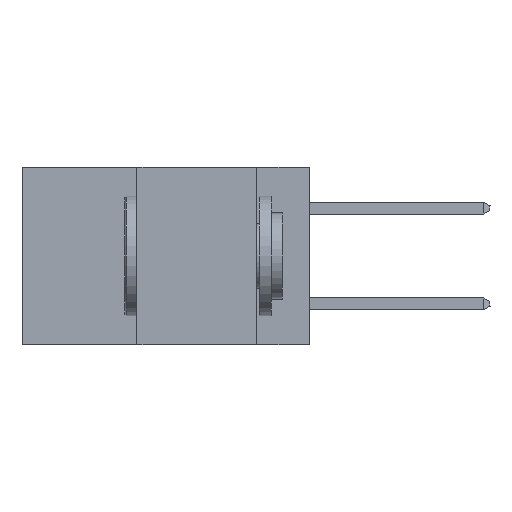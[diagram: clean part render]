
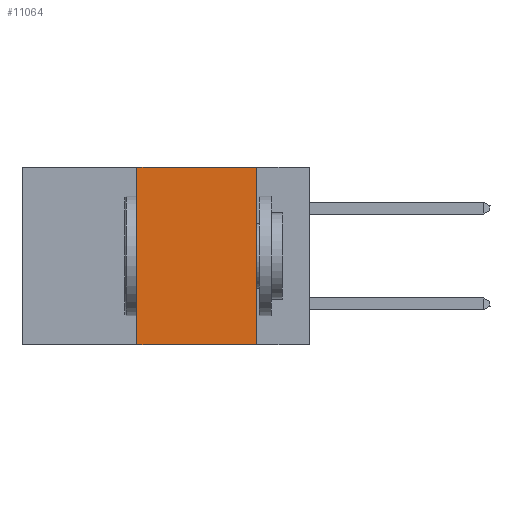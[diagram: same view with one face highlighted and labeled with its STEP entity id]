
A CAD part, left-side view. The second image highlights one B-rep face of the part: STEP entity #11064.
In plain terms, the highlighted planar face has unit normal (-1, 0, 0).
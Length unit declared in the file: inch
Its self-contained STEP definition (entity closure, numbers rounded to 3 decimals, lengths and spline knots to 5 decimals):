
#12 = LINE ( 'NONE', #3813, #2245 ) ;
#39 = CARTESIAN_POINT ( 'NONE',  ( 0., 0.36, 0. ) ) ;
#581 = DIRECTION ( 'NONE',  ( 0., 0., 1. ) ) ;
#1658 = LINE ( 'NONE', #6215, #11430 ) ;
#2245 = VECTOR ( 'NONE', #3767, 39.37008 ) ;
#2371 = ORIENTED_EDGE ( 'NONE', *, *, #6591, .F. ) ;
#3308 = ORIENTED_EDGE ( 'NONE', *, *, #4863, .F. ) ;
#3767 = DIRECTION ( 'NONE',  ( 0., 0., -1. ) ) ;
#3813 = CARTESIAN_POINT ( 'NONE',  ( 0., 0.11, 0. ) ) ;
#4354 = ORIENTED_EDGE ( 'NONE', *, *, #8156, .T. ) ;
#4803 = CARTESIAN_POINT ( 'NONE',  ( 0., 0.36, -0.37 ) ) ;
#4863 = EDGE_CURVE ( 'NONE', #8203, #6892, #10563, .T. ) ;
#5872 = EDGE_CURVE ( 'NONE', #9545, #8203, #1658, .T. ) ;
#6017 = DIRECTION ( 'NONE',  ( 1., 0., 0. ) ) ;
#6100 = DIRECTION ( 'NONE',  ( 0., 0., -1. ) ) ;
#6215 = CARTESIAN_POINT ( 'NONE',  ( 0., 0.36, 0. ) ) ;
#6272 = CARTESIAN_POINT ( 'NONE',  ( 0., 0.11, -0.37 ) ) ;
#6321 = AXIS2_PLACEMENT_3D ( 'NONE', #10754, #6017, #6100 ) ;
#6591 = EDGE_CURVE ( 'NONE', #6892, #11032, #12, .T. ) ;
#6824 = VECTOR ( 'NONE', #9668, 39.37008 ) ;
#6892 = VERTEX_POINT ( 'NONE', #11423 ) ;
#7393 = VECTOR ( 'NONE', #9389, 39.37008 ) ;
#7467 = FACE_OUTER_BOUND ( 'NONE', #9209, .T. ) ;
#8156 = EDGE_CURVE ( 'NONE', #9545, #11032, #8909, .T. ) ;
#8203 = VERTEX_POINT ( 'NONE', #39 ) ;
#8413 = CARTESIAN_POINT ( 'NONE',  ( 0., 0.6, 0. ) ) ;
#8909 = LINE ( 'NONE', #10421, #6824 ) ;
#9037 = ORIENTED_EDGE ( 'NONE', *, *, #5872, .F. ) ;
#9209 = EDGE_LOOP ( 'NONE', ( #2371, #3308, #9037, #4354 ) ) ;
#9389 = DIRECTION ( 'NONE',  ( 0., -1., 0. ) ) ;
#9545 = VERTEX_POINT ( 'NONE', #4803 ) ;
#9668 = DIRECTION ( 'NONE',  ( 0., -1., 0. ) ) ;
#9885 = PLANE ( 'NONE',  #6321 ) ;
#10421 = CARTESIAN_POINT ( 'NONE',  ( 0., 0.6, -0.37 ) ) ;
#10563 = LINE ( 'NONE', #8413, #7393 ) ;
#10754 = CARTESIAN_POINT ( 'NONE',  ( 0., 0.6, 0. ) ) ;
#11032 = VERTEX_POINT ( 'NONE', #6272 ) ;
#11064 = ADVANCED_FACE ( 'NONE', ( #7467 ), #9885, .F. ) ;
#11423 = CARTESIAN_POINT ( 'NONE',  ( 0., 0.11, 0. ) ) ;
#11430 = VECTOR ( 'NONE', #581, 39.37008 ) ;
